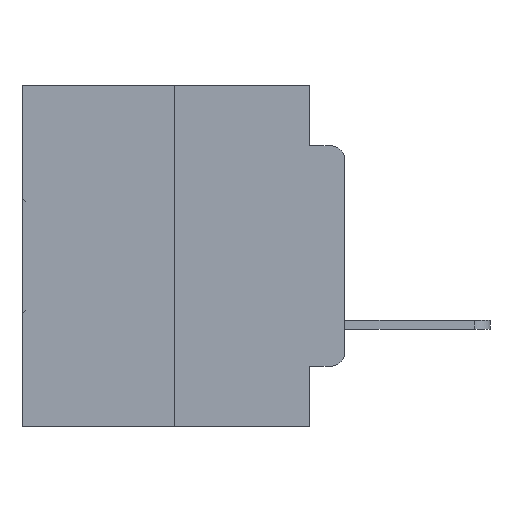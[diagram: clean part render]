
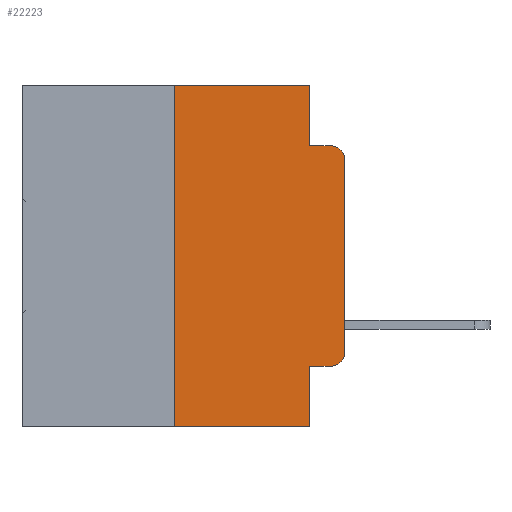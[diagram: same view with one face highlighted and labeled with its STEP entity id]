
A CAD part, left-side view. The second image highlights one B-rep face of the part: STEP entity #22223.
In plain terms, the highlighted planar face has unit normal (-1, 0, 0).
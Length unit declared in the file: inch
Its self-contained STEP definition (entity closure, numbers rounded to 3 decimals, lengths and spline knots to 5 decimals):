
#52 = VECTOR ( 'NONE', #5955, 39.37008 ) ;
#712 = VERTEX_POINT ( 'NONE', #10204 ) ;
#870 = AXIS2_PLACEMENT_3D ( 'NONE', #14103, #30312, #16429 ) ;
#1565 = EDGE_LOOP ( 'NONE', ( #6126, #14460, #20967, #29278, #14430, #26737, #8836, #16632, #19605, #11494 ) ) ;
#1726 = VERTEX_POINT ( 'NONE', #3296 ) ;
#1895 = DIRECTION ( 'NONE',  ( 0., 0., 1. ) ) ;
#2701 = EDGE_CURVE ( 'NONE', #28049, #12785, #23314, .T. ) ;
#3236 = VERTEX_POINT ( 'NONE', #26543 ) ;
#3296 = CARTESIAN_POINT ( 'NONE',  ( 0., 0.02, -0.4115 ) ) ;
#3403 = DIRECTION ( 'NONE',  ( 0., -1., 0. ) ) ;
#3614 = LINE ( 'NONE', #27242, #15718 ) ;
#4864 = CARTESIAN_POINT ( 'NONE',  ( 0., 0.473, 0. ) ) ;
#5955 = DIRECTION ( 'NONE',  ( 0., -1., 0. ) ) ;
#6053 = EDGE_CURVE ( 'NONE', #25718, #13020, #20202, .T. ) ;
#6126 = ORIENTED_EDGE ( 'NONE', *, *, #6680, .T. ) ;
#6268 = AXIS2_PLACEMENT_3D ( 'NONE', #12417, #28626, #14746 ) ;
#6523 = EDGE_CURVE ( 'NONE', #12785, #712, #7550, .T. ) ;
#6680 = EDGE_CURVE ( 'NONE', #29014, #20849, #3614, .T. ) ;
#6820 = DIRECTION ( 'NONE',  ( 0., -1., 0. ) ) ;
#7387 = DIRECTION ( 'NONE',  ( 0., 0., -1. ) ) ;
#7550 = LINE ( 'NONE', #28850, #52 ) ;
#8331 = EDGE_CURVE ( 'NONE', #20849, #3236, #9363, .T. ) ;
#8836 = ORIENTED_EDGE ( 'NONE', *, *, #24564, .T. ) ;
#9363 = CIRCLE ( 'NONE', #870, 0.02 ) ;
#10204 = CARTESIAN_POINT ( 'NONE',  ( 0., 0.051, 0. ) ) ;
#10682 = LINE ( 'NONE', #21729, #28522 ) ;
#11069 = LINE ( 'NONE', #20991, #24194 ) ;
#11415 = DIRECTION ( 'NONE',  ( 0., 0., -1. ) ) ;
#11494 = ORIENTED_EDGE ( 'NONE', *, *, #26526, .T. ) ;
#11611 = CARTESIAN_POINT ( 'NONE',  ( 0., 0.25, -0.5 ) ) ;
#12015 = CARTESIAN_POINT ( 'NONE',  ( 0., 0.25, 0. ) ) ;
#12417 = CARTESIAN_POINT ( 'NONE',  ( 0., 0.02, -0.3915 ) ) ;
#12575 = EDGE_CURVE ( 'NONE', #25718, #1726, #22954, .T. ) ;
#12785 = VERTEX_POINT ( 'NONE', #25431 ) ;
#13020 = VERTEX_POINT ( 'NONE', #27336 ) ;
#14103 = CARTESIAN_POINT ( 'NONE',  ( 0., 0.02, -0.1085 ) ) ;
#14430 = ORIENTED_EDGE ( 'NONE', *, *, #6523, .F. ) ;
#14460 = ORIENTED_EDGE ( 'NONE', *, *, #8331, .T. ) ;
#14746 = DIRECTION ( 'NONE',  ( 0., 0., -1. ) ) ;
#15718 = VECTOR ( 'NONE', #29597, 39.37008 ) ;
#15908 = CARTESIAN_POINT ( 'NONE',  ( 0., 0.051, -0.4115 ) ) ;
#16266 = EDGE_CURVE ( 'NONE', #29528, #3236, #10682, .T. ) ;
#16429 = DIRECTION ( 'NONE',  ( 0., 0., -1. ) ) ;
#16632 = ORIENTED_EDGE ( 'NONE', *, *, #6053, .F. ) ;
#16807 = CARTESIAN_POINT ( 'NONE',  ( 0., 0., -0.1085 ) ) ;
#17081 = DIRECTION ( 'NONE',  ( 0., -1., 0. ) ) ;
#17585 = CARTESIAN_POINT ( 'NONE',  ( 0., 0.051, -0.0885 ) ) ;
#18671 = VECTOR ( 'NONE', #11415, 39.37008 ) ;
#19392 = LINE ( 'NONE', #27567, #18671 ) ;
#19476 = VECTOR ( 'NONE', #24676, 39.37008 ) ;
#19605 = ORIENTED_EDGE ( 'NONE', *, *, #12575, .T. ) ;
#20202 = LINE ( 'NONE', #25209, #19476 ) ;
#20849 = VERTEX_POINT ( 'NONE', #16807 ) ;
#20967 = ORIENTED_EDGE ( 'NONE', *, *, #16266, .F. ) ;
#20991 = CARTESIAN_POINT ( 'NONE',  ( 0., 0.473, -0.5 ) ) ;
#21531 = DIRECTION ( 'NONE',  ( 1., 0., 0. ) ) ;
#21729 = CARTESIAN_POINT ( 'NONE',  ( 0., 0.051, -0.0885 ) ) ;
#22223 = ADVANCED_FACE ( 'NONE', ( #28034 ), #30688, .F. ) ;
#22520 = CARTESIAN_POINT ( 'NONE',  ( 0., 0.051, -0.4115 ) ) ;
#22521 = EDGE_CURVE ( 'NONE', #712, #29528, #19392, .T. ) ;
#22954 = LINE ( 'NONE', #22520, #28376 ) ;
#23314 = LINE ( 'NONE', #12015, #28725 ) ;
#24194 = VECTOR ( 'NONE', #6820, 39.37008 ) ;
#24564 = EDGE_CURVE ( 'NONE', #28049, #13020, #11069, .T. ) ;
#24676 = DIRECTION ( 'NONE',  ( 0., 0., -1. ) ) ;
#25120 = CIRCLE ( 'NONE', #6268, 0.02 ) ;
#25209 = CARTESIAN_POINT ( 'NONE',  ( 0., 0.051, 0. ) ) ;
#25431 = CARTESIAN_POINT ( 'NONE',  ( 0., 0.25, 0. ) ) ;
#25718 = VERTEX_POINT ( 'NONE', #15908 ) ;
#26526 = EDGE_CURVE ( 'NONE', #1726, #29014, #25120, .T. ) ;
#26543 = CARTESIAN_POINT ( 'NONE',  ( 0., 0.02, -0.0885 ) ) ;
#26737 = ORIENTED_EDGE ( 'NONE', *, *, #2701, .F. ) ;
#27218 = AXIS2_PLACEMENT_3D ( 'NONE', #4864, #21531, #7387 ) ;
#27242 = CARTESIAN_POINT ( 'NONE',  ( 0., 0., 0. ) ) ;
#27336 = CARTESIAN_POINT ( 'NONE',  ( 0., 0.051, -0.5 ) ) ;
#27567 = CARTESIAN_POINT ( 'NONE',  ( 0., 0.051, 0. ) ) ;
#28034 = FACE_OUTER_BOUND ( 'NONE', #1565, .T. ) ;
#28049 = VERTEX_POINT ( 'NONE', #11611 ) ;
#28376 = VECTOR ( 'NONE', #3403, 39.37008 ) ;
#28522 = VECTOR ( 'NONE', #17081, 39.37008 ) ;
#28610 = CARTESIAN_POINT ( 'NONE',  ( 0., 0., -0.3915 ) ) ;
#28626 = DIRECTION ( 'NONE',  ( -1., 0., 0. ) ) ;
#28725 = VECTOR ( 'NONE', #1895, 39.37008 ) ;
#28850 = CARTESIAN_POINT ( 'NONE',  ( 0., 0.473, 0. ) ) ;
#29014 = VERTEX_POINT ( 'NONE', #28610 ) ;
#29278 = ORIENTED_EDGE ( 'NONE', *, *, #22521, .F. ) ;
#29528 = VERTEX_POINT ( 'NONE', #17585 ) ;
#29597 = DIRECTION ( 'NONE',  ( 0., 0., 1. ) ) ;
#30312 = DIRECTION ( 'NONE',  ( -1., 0., 0. ) ) ;
#30688 = PLANE ( 'NONE',  #27218 ) ;
